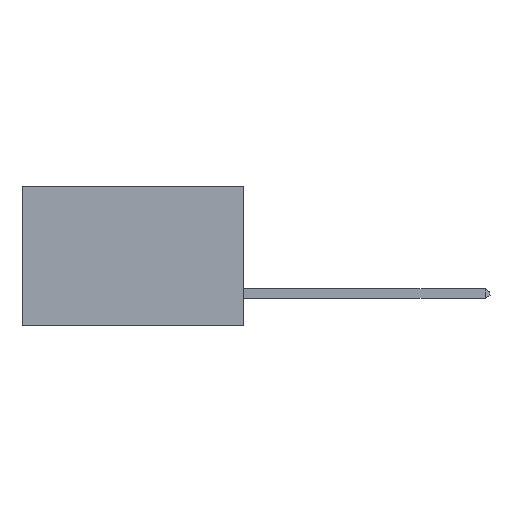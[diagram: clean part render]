
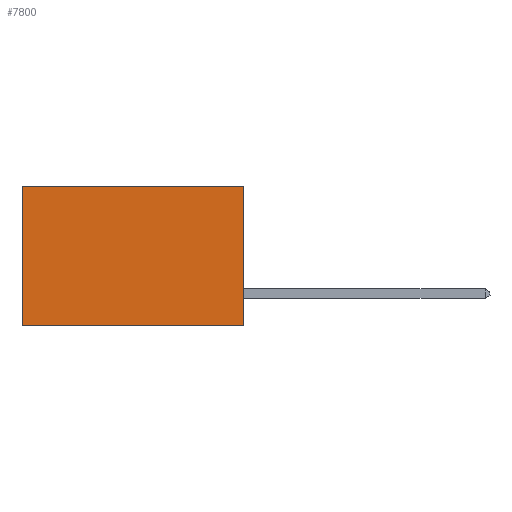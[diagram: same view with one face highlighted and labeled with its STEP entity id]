
A CAD part, left-side view. The second image highlights one B-rep face of the part: STEP entity #7800.
In plain terms, the highlighted planar face has unit normal (-1, 0, 0).
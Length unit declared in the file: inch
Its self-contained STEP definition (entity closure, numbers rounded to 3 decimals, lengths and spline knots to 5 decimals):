
#334 = ORIENTED_EDGE ( 'NONE', *, *, #12884, .T. ) ;
#2126 = VECTOR ( 'NONE', #11530, 39.37008 ) ;
#2414 = VERTEX_POINT ( 'NONE', #6674 ) ;
#2978 = EDGE_LOOP ( 'NONE', ( #334, #12858, #10387, #12487 ) ) ;
#2982 = VECTOR ( 'NONE', #11064, 39.37008 ) ;
#3348 = LINE ( 'NONE', #13505, #2982 ) ;
#4276 = FACE_OUTER_BOUND ( 'NONE', #2978, .T. ) ;
#4586 = LINE ( 'NONE', #12117, #2126 ) ;
#4976 = DIRECTION ( 'NONE',  ( 0., 0., -1. ) ) ;
#6052 = VECTOR ( 'NONE', #4976, 39.37008 ) ;
#6365 = DIRECTION ( 'NONE',  ( 0., 0., -1. ) ) ;
#6674 = CARTESIAN_POINT ( 'NONE',  ( 0.277, 0.59, -0.37 ) ) ;
#7552 = DIRECTION ( 'NONE',  ( 0., 1., 0. ) ) ;
#7709 = CARTESIAN_POINT ( 'NONE',  ( 0.277, 0., -0.37 ) ) ;
#7800 = ADVANCED_FACE ( 'NONE', ( #4276 ), #13259, .F. ) ;
#8219 = VERTEX_POINT ( 'NONE', #7709 ) ;
#8484 = CARTESIAN_POINT ( 'NONE',  ( 0.277, 0., -0.37 ) ) ;
#8582 = VERTEX_POINT ( 'NONE', #13755 ) ;
#8721 = CARTESIAN_POINT ( 'NONE',  ( 0.277, 0., 0. ) ) ;
#9535 = DIRECTION ( 'NONE',  ( 1., 0., 0. ) ) ;
#10191 = EDGE_CURVE ( 'NONE', #8219, #2414, #4586, .T. ) ;
#10387 = ORIENTED_EDGE ( 'NONE', *, *, #13379, .F. ) ;
#11064 = DIRECTION ( 'NONE',  ( 0., 0., -1. ) ) ;
#11530 = DIRECTION ( 'NONE',  ( 0., 1., 0. ) ) ;
#11846 = VERTEX_POINT ( 'NONE', #12758 ) ;
#11995 = LINE ( 'NONE', #8484, #6052 ) ;
#12117 = CARTESIAN_POINT ( 'NONE',  ( 0.277, 0., -0.37 ) ) ;
#12248 = EDGE_CURVE ( 'NONE', #8582, #11846, #15616, .T. ) ;
#12322 = VECTOR ( 'NONE', #7552, 39.37008 ) ;
#12398 = CARTESIAN_POINT ( 'NONE',  ( 0.277, 0., -0.37 ) ) ;
#12487 = ORIENTED_EDGE ( 'NONE', *, *, #12248, .T. ) ;
#12758 = CARTESIAN_POINT ( 'NONE',  ( 0.277, 0.59, 0. ) ) ;
#12858 = ORIENTED_EDGE ( 'NONE', *, *, #10191, .F. ) ;
#12884 = EDGE_CURVE ( 'NONE', #11846, #2414, #3348, .T. ) ;
#13259 = PLANE ( 'NONE',  #14238 ) ;
#13379 = EDGE_CURVE ( 'NONE', #8582, #8219, #11995, .T. ) ;
#13505 = CARTESIAN_POINT ( 'NONE',  ( 0.277, 0.59, -0.37 ) ) ;
#13755 = CARTESIAN_POINT ( 'NONE',  ( 0.277, 0., 0. ) ) ;
#14238 = AXIS2_PLACEMENT_3D ( 'NONE', #12398, #9535, #6365 ) ;
#15616 = LINE ( 'NONE', #8721, #12322 ) ;
